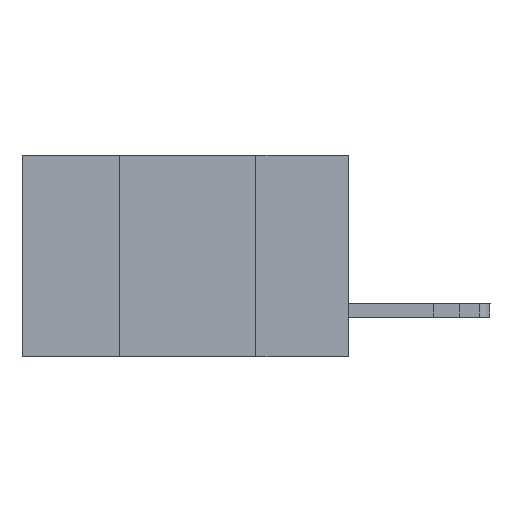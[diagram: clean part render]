
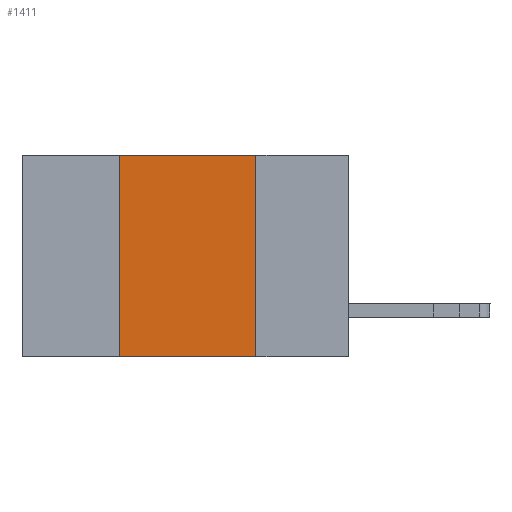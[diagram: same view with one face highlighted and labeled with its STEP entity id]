
A CAD part, left-side view. The second image highlights one B-rep face of the part: STEP entity #1411.
In plain terms, the highlighted planar face has unit normal (-1, 0, 0).
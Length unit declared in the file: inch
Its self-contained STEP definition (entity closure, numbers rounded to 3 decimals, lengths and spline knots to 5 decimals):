
#350 = CARTESIAN_POINT ( 'NONE',  ( 0., 0.6, 0. ) ) ;
#746 = CARTESIAN_POINT ( 'NONE',  ( 0., 0.42, 0. ) ) ;
#1163 = CARTESIAN_POINT ( 'NONE',  ( 0., 0.6, -0.37 ) ) ;
#1304 = VECTOR ( 'NONE', #2355, 39.37008 ) ;
#1411 = ADVANCED_FACE ( 'NONE', ( #6761 ), #9699, .F. ) ;
#1415 = CARTESIAN_POINT ( 'NONE',  ( 0., 0.17, -0.37 ) ) ;
#1928 = VERTEX_POINT ( 'NONE', #746 ) ;
#2355 = DIRECTION ( 'NONE',  ( 0., 0., -1. ) ) ;
#2654 = VECTOR ( 'NONE', #5305, 39.37008 ) ;
#2788 = CARTESIAN_POINT ( 'NONE',  ( 0., 0.17, -0.37 ) ) ;
#2804 = LINE ( 'NONE', #3008, #5423 ) ;
#2996 = EDGE_CURVE ( 'NONE', #1928, #3483, #4167, .T. ) ;
#3008 = CARTESIAN_POINT ( 'NONE',  ( 0., 0.42, -0.37 ) ) ;
#3365 = ORIENTED_EDGE ( 'NONE', *, *, #7629, .T. ) ;
#3483 = VERTEX_POINT ( 'NONE', #9395 ) ;
#3579 = LINE ( 'NONE', #1415, #1304 ) ;
#3612 = EDGE_CURVE ( 'NONE', #3483, #6781, #3579, .T. ) ;
#4167 = LINE ( 'NONE', #8326, #8253 ) ;
#4913 = VERTEX_POINT ( 'NONE', #9859 ) ;
#5305 = DIRECTION ( 'NONE',  ( 0., -1., 0. ) ) ;
#5423 = VECTOR ( 'NONE', #7182, 39.37008 ) ;
#6040 = AXIS2_PLACEMENT_3D ( 'NONE', #350, #12796, #6628 ) ;
#6061 = ORIENTED_EDGE ( 'NONE', *, *, #2996, .F. ) ;
#6628 = DIRECTION ( 'NONE',  ( 0., 0., -1. ) ) ;
#6761 = FACE_OUTER_BOUND ( 'NONE', #11181, .T. ) ;
#6781 = VERTEX_POINT ( 'NONE', #2788 ) ;
#7182 = DIRECTION ( 'NONE',  ( 0., 0., 1. ) ) ;
#7629 = EDGE_CURVE ( 'NONE', #4913, #6781, #10502, .T. ) ;
#8253 = VECTOR ( 'NONE', #12465, 39.37008 ) ;
#8326 = CARTESIAN_POINT ( 'NONE',  ( 0., 0.6, 0. ) ) ;
#9023 = EDGE_CURVE ( 'NONE', #4913, #1928, #2804, .T. ) ;
#9395 = CARTESIAN_POINT ( 'NONE',  ( 0., 0.17, 0. ) ) ;
#9699 = PLANE ( 'NONE',  #6040 ) ;
#9859 = CARTESIAN_POINT ( 'NONE',  ( 0., 0.42, -0.37 ) ) ;
#10502 = LINE ( 'NONE', #1163, #2654 ) ;
#11181 = EDGE_LOOP ( 'NONE', ( #11182, #6061, #12997, #3365 ) ) ;
#11182 = ORIENTED_EDGE ( 'NONE', *, *, #3612, .F. ) ;
#12465 = DIRECTION ( 'NONE',  ( 0., -1., 0. ) ) ;
#12796 = DIRECTION ( 'NONE',  ( 1., 0., 0. ) ) ;
#12997 = ORIENTED_EDGE ( 'NONE', *, *, #9023, .F. ) ;
